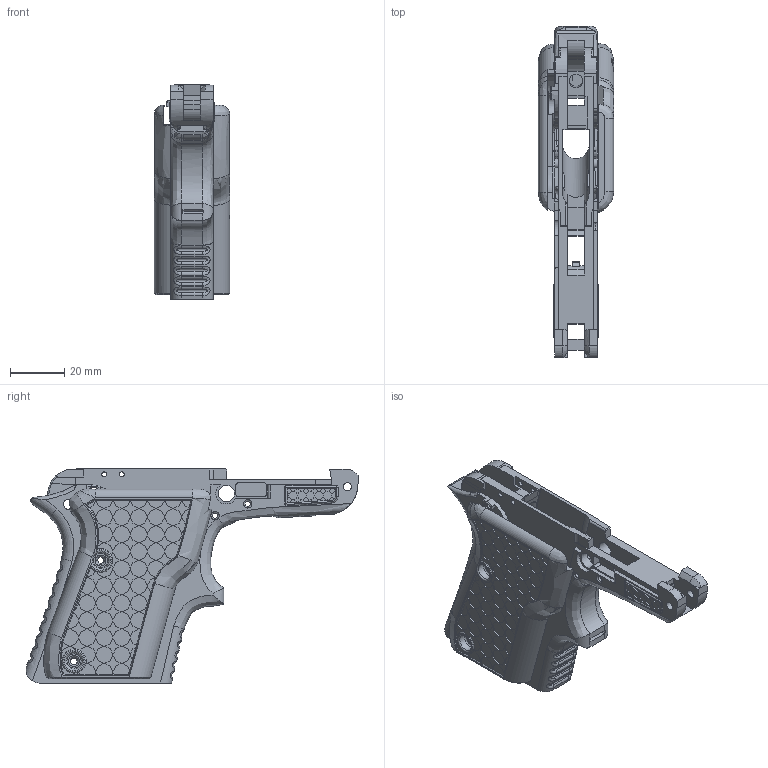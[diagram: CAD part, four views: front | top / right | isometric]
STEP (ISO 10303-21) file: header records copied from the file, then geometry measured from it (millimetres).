
FILE_DESCRIPTION(/* description */ (''),/* implementation_level */ '2;1');
FILE_NAME(/* name */ '21a-export-frame-and-grips.step',/* time_stamp */ '2021-11-09T19:53:41-08:00',/* author */ (''),/* organization */ (''),/* preprocessor_version */ 'ST-DEVELOPER v18.1',/* originating_system */ 'Autodesk Translation Framework v10.10.0.1391',/* authorisation */ '');
FILE_SCHEMA (('AUTOMOTIVE_DESIGN { 1 0 10303 214 3 1 1 }'));
Length unit declared in the file: millimetre
Products named in the file (4): bobkatz-bobcat-21a-final-cleanedup; 21a-frame-final; Grip-L-Final; Grip-R-Final
Assembly tree (3 placements, depth 2):
  bobkatz-bobcat-21a-final-cleanedup
    21a-frame-final
    Grip-L-Final
    Grip-R-Final
Bounding box: 27.75 x 122.46 x 78.94 mm (x, y, z)
Volume: 67669.3 mm3; surface area: 42220.3 mm2
Topology: 3 solids, 3 shells, 2855 faces, 7945 edges, 5176 vertices
Faces by surface type: plane 1390, bspline 1132, cylinder 276, torus 33, cone 22, sphere 2
Full cylindrical faces by diameter (mm): 1.8 x4, 2.05 x2, 2.1 x2, 2.14 x2, 2.5 x3, 2.98 x2, 3 x6, 3.8 x4, 5 x1, 5.5 x1, 6.1 x2, 6.2 x4, 7.2 x1, 8.2 x1, 8.4 x1, 8.7 x1, 18.002 x1
Entity records: 117896 total; most frequent: CARTESIAN_POINT 52091, ORIENTED_EDGE 15866, DIRECTION 9774, EDGE_CURVE 7933, VERTEX_POINT 5176, LINE 4816, VECTOR 4816, EDGE_LOOP 3025
